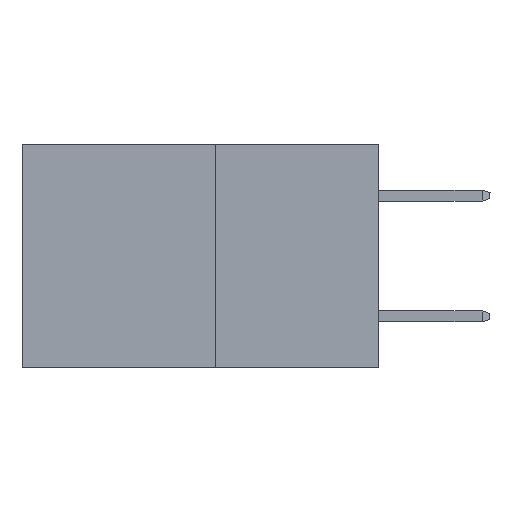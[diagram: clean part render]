
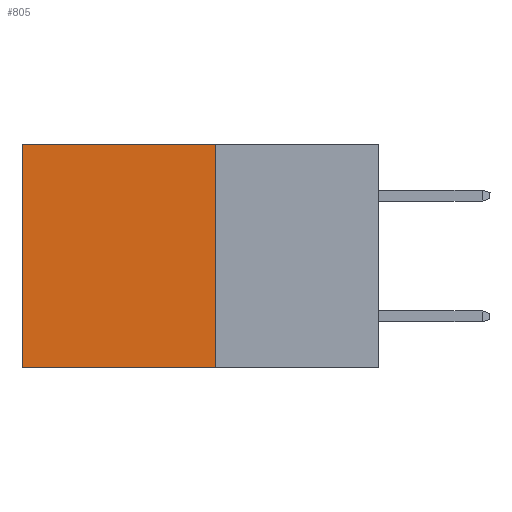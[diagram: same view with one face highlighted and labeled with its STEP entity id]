
A CAD part, left-side view. The second image highlights one B-rep face of the part: STEP entity #805.
In plain terms, the highlighted planar face has unit normal (-1, 0, 0).
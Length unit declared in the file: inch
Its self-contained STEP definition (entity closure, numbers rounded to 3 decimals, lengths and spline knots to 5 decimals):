
#805 = ADVANCED_FACE ( 'NONE', ( #18269 ), #7118, .F. ) ;
#920 = CARTESIAN_POINT ( 'NONE',  ( 0.277, 0.27, -0.37 ) ) ;
#935 = ORIENTED_EDGE ( 'NONE', *, *, #20666, .T. ) ;
#1918 = DIRECTION ( 'NONE',  ( 0., 0., -1. ) ) ;
#4756 = CARTESIAN_POINT ( 'NONE',  ( 0.277, 0.59, 0. ) ) ;
#4824 = LINE ( 'NONE', #23916, #27562 ) ;
#5208 = VERTEX_POINT ( 'NONE', #4756 ) ;
#6859 = LINE ( 'NONE', #13438, #17234 ) ;
#7118 = PLANE ( 'NONE',  #9079 ) ;
#7318 = DIRECTION ( 'NONE',  ( 0., 1., 0. ) ) ;
#8946 = EDGE_CURVE ( 'NONE', #5208, #25193, #4824, .T. ) ;
#9079 = AXIS2_PLACEMENT_3D ( 'NONE', #26664, #11242, #20371 ) ;
#9349 = ORIENTED_EDGE ( 'NONE', *, *, #20774, .F. ) ;
#10314 = VERTEX_POINT ( 'NONE', #17052 ) ;
#10557 = CARTESIAN_POINT ( 'NONE',  ( 0.277, 0.59, -0.37 ) ) ;
#11242 = DIRECTION ( 'NONE',  ( 1., 0., 0. ) ) ;
#12480 = EDGE_CURVE ( 'NONE', #10314, #25019, #25667, .T. ) ;
#12495 = CARTESIAN_POINT ( 'NONE',  ( 0.277, 0.27, -0.37 ) ) ;
#13438 = CARTESIAN_POINT ( 'NONE',  ( 0.277, 0.27, 0. ) ) ;
#14432 = VECTOR ( 'NONE', #7318, 39.37008 ) ;
#14655 = DIRECTION ( 'NONE',  ( 0., 0., -1. ) ) ;
#17052 = CARTESIAN_POINT ( 'NONE',  ( 0.277, 0.27, 0. ) ) ;
#17073 = ORIENTED_EDGE ( 'NONE', *, *, #8946, .T. ) ;
#17234 = VECTOR ( 'NONE', #26556, 39.37008 ) ;
#18269 = FACE_OUTER_BOUND ( 'NONE', #19753, .T. ) ;
#19686 = ORIENTED_EDGE ( 'NONE', *, *, #12480, .F. ) ;
#19753 = EDGE_LOOP ( 'NONE', ( #17073, #9349, #19686, #935 ) ) ;
#20371 = DIRECTION ( 'NONE',  ( 0., 0., -1. ) ) ;
#20544 = CARTESIAN_POINT ( 'NONE',  ( 0.277, 0.27, -0.37 ) ) ;
#20666 = EDGE_CURVE ( 'NONE', #10314, #5208, #6859, .T. ) ;
#20774 = EDGE_CURVE ( 'NONE', #25019, #25193, #25431, .T. ) ;
#23916 = CARTESIAN_POINT ( 'NONE',  ( 0.277, 0.59, -0.37 ) ) ;
#24963 = VECTOR ( 'NONE', #14655, 39.37008 ) ;
#25019 = VERTEX_POINT ( 'NONE', #920 ) ;
#25193 = VERTEX_POINT ( 'NONE', #10557 ) ;
#25431 = LINE ( 'NONE', #20544, #14432 ) ;
#25667 = LINE ( 'NONE', #12495, #24963 ) ;
#26556 = DIRECTION ( 'NONE',  ( 0., 1., 0. ) ) ;
#26664 = CARTESIAN_POINT ( 'NONE',  ( 0.277, 0.27, -0.37 ) ) ;
#27562 = VECTOR ( 'NONE', #1918, 39.37008 ) ;
